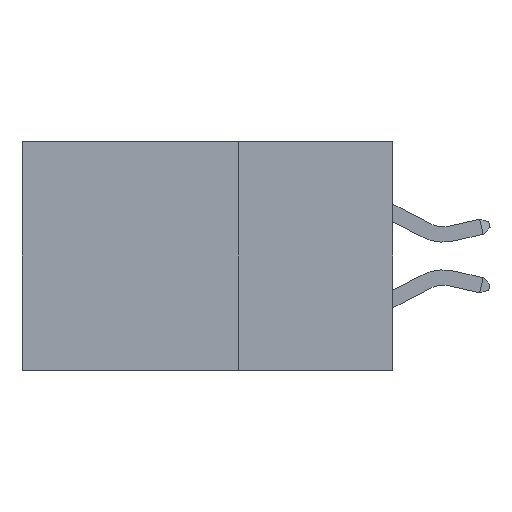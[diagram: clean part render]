
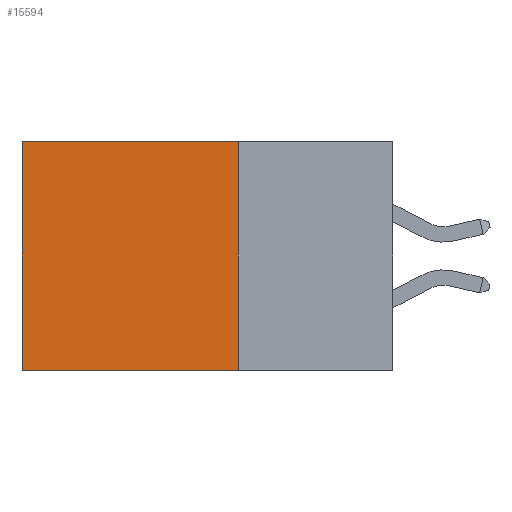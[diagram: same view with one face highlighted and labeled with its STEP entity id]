
A CAD part, left-side view. The second image highlights one B-rep face of the part: STEP entity #15594.
In plain terms, the highlighted planar face has unit normal (-1, 0, 0).
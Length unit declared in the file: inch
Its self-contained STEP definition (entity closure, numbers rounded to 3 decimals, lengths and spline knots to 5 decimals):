
#1476 = ORIENTED_EDGE ( 'NONE', *, *, #11541, .F. ) ;
#1519 = DIRECTION ( 'NONE',  ( 1., 0., 0. ) ) ;
#2364 = FACE_OUTER_BOUND ( 'NONE', #6283, .T. ) ;
#2458 = EDGE_CURVE ( 'NONE', #16118, #4469, #6231, .T. ) ;
#3014 = VERTEX_POINT ( 'NONE', #3431 ) ;
#3431 = CARTESIAN_POINT ( 'NONE',  ( 0.2875, 0.25, -0.37 ) ) ;
#3964 = VECTOR ( 'NONE', #21046, 39.37008 ) ;
#3966 = VECTOR ( 'NONE', #5973, 39.37008 ) ;
#4469 = VERTEX_POINT ( 'NONE', #12893 ) ;
#5289 = CARTESIAN_POINT ( 'NONE',  ( 0.2875, 0.25, 0. ) ) ;
#5480 = PLANE ( 'NONE',  #14556 ) ;
#5973 = DIRECTION ( 'NONE',  ( 0., 1., 0. ) ) ;
#6231 = LINE ( 'NONE', #8427, #3964 ) ;
#6283 = EDGE_LOOP ( 'NONE', ( #11737, #1476, #13516, #22288 ) ) ;
#7263 = CARTESIAN_POINT ( 'NONE',  ( 0.2875, 0.25, -0.37 ) ) ;
#8427 = CARTESIAN_POINT ( 'NONE',  ( 0.2875, 0.25, 0. ) ) ;
#8768 = CARTESIAN_POINT ( 'NONE',  ( 0.2875, 0.6, 0. ) ) ;
#9617 = VECTOR ( 'NONE', #19895, 39.37008 ) ;
#10029 = LINE ( 'NONE', #8768, #22196 ) ;
#11541 = EDGE_CURVE ( 'NONE', #3014, #19876, #19561, .T. ) ;
#11737 = ORIENTED_EDGE ( 'NONE', *, *, #18805, .T. ) ;
#12597 = CARTESIAN_POINT ( 'NONE',  ( 0.2875, 0.25, 0. ) ) ;
#12893 = CARTESIAN_POINT ( 'NONE',  ( 0.2875, 0.6, 0. ) ) ;
#13516 = ORIENTED_EDGE ( 'NONE', *, *, #22015, .F. ) ;
#14418 = LINE ( 'NONE', #12597, #9617 ) ;
#14556 = AXIS2_PLACEMENT_3D ( 'NONE', #21583, #1519, #16057 ) ;
#15498 = CARTESIAN_POINT ( 'NONE',  ( 0.2875, 0.6, -0.37 ) ) ;
#15594 = ADVANCED_FACE ( 'NONE', ( #2364 ), #5480, .F. ) ;
#16057 = DIRECTION ( 'NONE',  ( 0., 0., -1. ) ) ;
#16118 = VERTEX_POINT ( 'NONE', #5289 ) ;
#18805 = EDGE_CURVE ( 'NONE', #4469, #19876, #10029, .T. ) ;
#19561 = LINE ( 'NONE', #7263, #3966 ) ;
#19876 = VERTEX_POINT ( 'NONE', #15498 ) ;
#19895 = DIRECTION ( 'NONE',  ( 0., 0., -1. ) ) ;
#21046 = DIRECTION ( 'NONE',  ( 0., 1., 0. ) ) ;
#21323 = DIRECTION ( 'NONE',  ( 0., 0., -1. ) ) ;
#21583 = CARTESIAN_POINT ( 'NONE',  ( 0.2875, 0.25, 0. ) ) ;
#22015 = EDGE_CURVE ( 'NONE', #16118, #3014, #14418, .T. ) ;
#22196 = VECTOR ( 'NONE', #21323, 39.37008 ) ;
#22288 = ORIENTED_EDGE ( 'NONE', *, *, #2458, .T. ) ;
